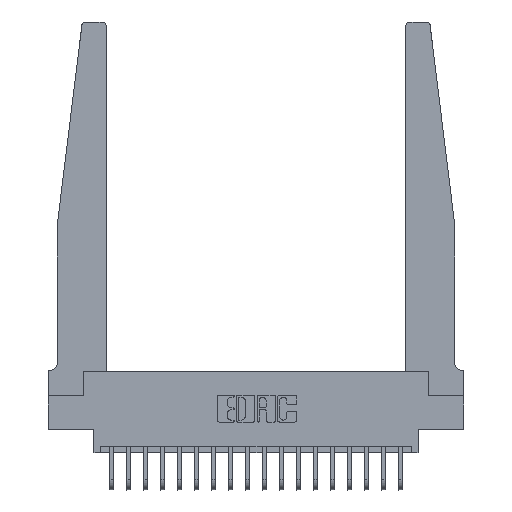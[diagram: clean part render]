
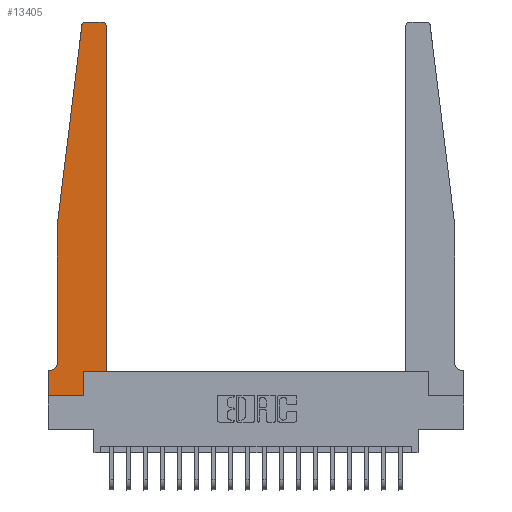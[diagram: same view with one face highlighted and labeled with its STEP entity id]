
A CAD part, top view. The second image highlights one B-rep face of the part: STEP entity #13405.
In plain terms, the highlighted planar face has unit normal (0, 0, 1).
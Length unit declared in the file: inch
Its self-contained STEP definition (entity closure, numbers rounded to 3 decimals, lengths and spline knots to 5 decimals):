
#193 = DIRECTION ( 'NONE',  ( 0., 0., 1. ) ) ;
#352 = VERTEX_POINT ( 'NONE', #1040 ) ;
#524 = VECTOR ( 'NONE', #5617, 39.37008 ) ;
#739 = CIRCLE ( 'NONE', #12512, 0.03 ) ;
#1040 = CARTESIAN_POINT ( 'NONE',  ( 0.425, 2.72, 0.37 ) ) ;
#1185 = DIRECTION ( 'NONE',  ( -1., 0., 0. ) ) ;
#1359 = DIRECTION ( 'NONE',  ( 1., 0., 0. ) ) ;
#1494 = ORIENTED_EDGE ( 'NONE', *, *, #2830, .T. ) ;
#1661 = DIRECTION ( 'NONE',  ( 0., 1., 0. ) ) ;
#2019 = ORIENTED_EDGE ( 'NONE', *, *, #5529, .T. ) ;
#2182 = CARTESIAN_POINT ( 'NONE',  ( 0.2605, 0., 0.37 ) ) ;
#2326 = CARTESIAN_POINT ( 'NONE',  ( 0., 0., 0.37 ) ) ;
#2641 = CARTESIAN_POINT ( 'NONE',  ( 0.015, 0.1875, 0.37 ) ) ;
#2776 = VECTOR ( 'NONE', #10563, 39.37008 ) ;
#2830 = EDGE_CURVE ( 'NONE', #15628, #21387, #20322, .T. ) ;
#3011 = LINE ( 'NONE', #6701, #21854 ) ;
#3212 = ORIENTED_EDGE ( 'NONE', *, *, #11131, .T. ) ;
#3809 = VERTEX_POINT ( 'NONE', #6713 ) ;
#3873 = CARTESIAN_POINT ( 'NONE',  ( 0., 0.1875, 0.37 ) ) ;
#4054 = CARTESIAN_POINT ( 'NONE',  ( 0.425, 0.18, 0.37 ) ) ;
#4357 = CARTESIAN_POINT ( 'NONE',  ( 0.395, 2.72, 0.37 ) ) ;
#4691 = EDGE_CURVE ( 'NONE', #8850, #16879, #18824, .T. ) ;
#5171 = CARTESIAN_POINT ( 'NONE',  ( 0., 0.1875, 0.37 ) ) ;
#5229 = ORIENTED_EDGE ( 'NONE', *, *, #12447, .T. ) ;
#5368 = CARTESIAN_POINT ( 'NONE',  ( 0.425, 0.18, 0.37 ) ) ;
#5446 = DIRECTION ( 'NONE',  ( 1., 0., 0. ) ) ;
#5529 = EDGE_CURVE ( 'NONE', #9274, #3809, #3011, .T. ) ;
#5617 = DIRECTION ( 'NONE',  ( -1., 0., 0. ) ) ;
#5804 = DIRECTION ( 'NONE',  ( -0.122, -0.992, 0. ) ) ;
#5879 = CARTESIAN_POINT ( 'NONE',  ( 0., 0., 0.37 ) ) ;
#5976 = DIRECTION ( 'NONE',  ( 0., 1., 0. ) ) ;
#6336 = VECTOR ( 'NONE', #7044, 39.37008 ) ;
#6351 = VECTOR ( 'NONE', #5976, 39.37008 ) ;
#6701 = CARTESIAN_POINT ( 'NONE',  ( 0.2605, 0.18, 0.37 ) ) ;
#6713 = CARTESIAN_POINT ( 'NONE',  ( 0.2605, 0.18, 0.37 ) ) ;
#6799 = VERTEX_POINT ( 'NONE', #2641 ) ;
#7044 = DIRECTION ( 'NONE',  ( 0., -1., 0. ) ) ;
#7048 = CARTESIAN_POINT ( 'NONE',  ( 0.25, 2.75, 0.37 ) ) ;
#7054 = EDGE_LOOP ( 'NONE', ( #13922, #5229, #18805, #1494, #21641, #3212, #13097, #16785, #2019, #14179, #14678, #8646 ) ) ;
#7327 = DIRECTION ( 'NONE',  ( 1., 0., 0. ) ) ;
#7843 = EDGE_CURVE ( 'NONE', #21387, #6799, #19348, .T. ) ;
#8334 = VERTEX_POINT ( 'NONE', #5171 ) ;
#8646 = ORIENTED_EDGE ( 'NONE', *, *, #18179, .T. ) ;
#8850 = VERTEX_POINT ( 'NONE', #10936 ) ;
#9012 = DIRECTION ( 'NONE',  ( -1., 0., 0. ) ) ;
#9274 = VERTEX_POINT ( 'NONE', #2182 ) ;
#9733 = CARTESIAN_POINT ( 'NONE',  ( 0.065, 1.25, 0.37 ) ) ;
#10179 = EDGE_CURVE ( 'NONE', #13621, #9274, #14346, .T. ) ;
#10535 = CARTESIAN_POINT ( 'NONE',  ( 0.27653, 2.72, 0.37 ) ) ;
#10563 = DIRECTION ( 'NONE',  ( 0., -1., 0. ) ) ;
#10910 = LINE ( 'NONE', #17715, #2776 ) ;
#10936 = CARTESIAN_POINT ( 'NONE',  ( 0.395, 2.75, 0.37 ) ) ;
#11131 = EDGE_CURVE ( 'NONE', #6799, #8334, #14093, .T. ) ;
#11653 = VECTOR ( 'NONE', #5804, 39.37008 ) ;
#11809 = CARTESIAN_POINT ( 'NONE',  ( 0.065, 0.2375, 0.37 ) ) ;
#12377 = EDGE_CURVE ( 'NONE', #20386, #15628, #14172, .T. ) ;
#12447 = EDGE_CURVE ( 'NONE', #16879, #20386, #21626, .T. ) ;
#12493 = FACE_OUTER_BOUND ( 'NONE', #7054, .T. ) ;
#12512 = AXIS2_PLACEMENT_3D ( 'NONE', #4357, #16305, #1359 ) ;
#12712 = AXIS2_PLACEMENT_3D ( 'NONE', #10535, #193, #13814 ) ;
#12960 = EDGE_CURVE ( 'NONE', #3809, #18482, #13176, .T. ) ;
#12969 = AXIS2_PLACEMENT_3D ( 'NONE', #21414, #13261, #1185 ) ;
#13042 = CARTESIAN_POINT ( 'NONE',  ( 0.24675, 2.72367, 0.37 ) ) ;
#13097 = ORIENTED_EDGE ( 'NONE', *, *, #20130, .T. ) ;
#13176 = LINE ( 'NONE', #18151, #16613 ) ;
#13261 = DIRECTION ( 'NONE',  ( 0., 0., -1. ) ) ;
#13298 = CARTESIAN_POINT ( 'NONE',  ( 0.065, 1.25, 0.37 ) ) ;
#13405 = ADVANCED_FACE ( 'NONE', ( #12493 ), #20835, .T. ) ;
#13621 = VERTEX_POINT ( 'NONE', #2326 ) ;
#13814 = DIRECTION ( 'NONE',  ( 1., 0., 0. ) ) ;
#13865 = CARTESIAN_POINT ( 'NONE',  ( 0.27653, 2.75, 0.37 ) ) ;
#13922 = ORIENTED_EDGE ( 'NONE', *, *, #4691, .T. ) ;
#14093 = LINE ( 'NONE', #14201, #524 ) ;
#14172 = LINE ( 'NONE', #20981, #11653 ) ;
#14179 = ORIENTED_EDGE ( 'NONE', *, *, #12960, .T. ) ;
#14201 = CARTESIAN_POINT ( 'NONE',  ( 0.065, 0.1875, 0.37 ) ) ;
#14346 = LINE ( 'NONE', #5879, #21935 ) ;
#14678 = ORIENTED_EDGE ( 'NONE', *, *, #16263, .T. ) ;
#15536 = AXIS2_PLACEMENT_3D ( 'NONE', #3873, #15803, #5446 ) ;
#15628 = VERTEX_POINT ( 'NONE', #13298 ) ;
#15803 = DIRECTION ( 'NONE',  ( 0., 0., 1. ) ) ;
#16263 = EDGE_CURVE ( 'NONE', #18482, #352, #21047, .T. ) ;
#16305 = DIRECTION ( 'NONE',  ( 0., 0., 1. ) ) ;
#16613 = VECTOR ( 'NONE', #18486, 39.37008 ) ;
#16785 = ORIENTED_EDGE ( 'NONE', *, *, #10179, .T. ) ;
#16879 = VERTEX_POINT ( 'NONE', #13865 ) ;
#17715 = CARTESIAN_POINT ( 'NONE',  ( 0., 0., 0.37 ) ) ;
#18151 = CARTESIAN_POINT ( 'NONE',  ( 0.425, 0.18, 0.37 ) ) ;
#18179 = EDGE_CURVE ( 'NONE', #352, #8850, #739, .T. ) ;
#18482 = VERTEX_POINT ( 'NONE', #5368 ) ;
#18486 = DIRECTION ( 'NONE',  ( 1., 0., 0. ) ) ;
#18805 = ORIENTED_EDGE ( 'NONE', *, *, #12377, .T. ) ;
#18824 = LINE ( 'NONE', #7048, #20355 ) ;
#19348 = CIRCLE ( 'NONE', #12969, 0.05 ) ;
#20130 = EDGE_CURVE ( 'NONE', #8334, #13621, #10910, .T. ) ;
#20322 = LINE ( 'NONE', #9733, #6336 ) ;
#20355 = VECTOR ( 'NONE', #9012, 39.37008 ) ;
#20386 = VERTEX_POINT ( 'NONE', #13042 ) ;
#20835 = PLANE ( 'NONE',  #15536 ) ;
#20981 = CARTESIAN_POINT ( 'NONE',  ( 0.065, 1.25, 0.37 ) ) ;
#21047 = LINE ( 'NONE', #4054, #6351 ) ;
#21387 = VERTEX_POINT ( 'NONE', #11809 ) ;
#21414 = CARTESIAN_POINT ( 'NONE',  ( 0.015, 0.2375, 0.37 ) ) ;
#21626 = CIRCLE ( 'NONE', #12712, 0.03 ) ;
#21641 = ORIENTED_EDGE ( 'NONE', *, *, #7843, .T. ) ;
#21854 = VECTOR ( 'NONE', #1661, 39.37008 ) ;
#21935 = VECTOR ( 'NONE', #7327, 39.37008 ) ;
